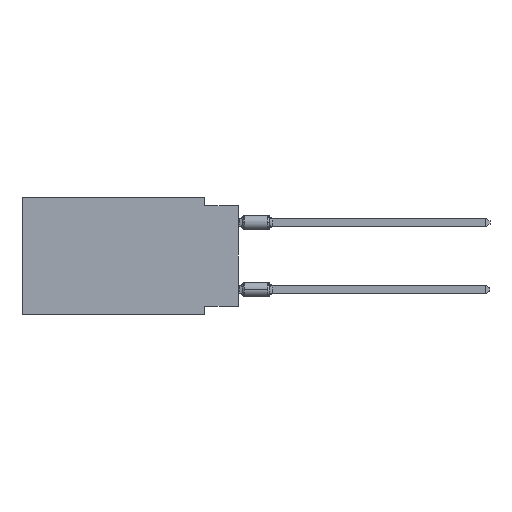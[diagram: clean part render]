
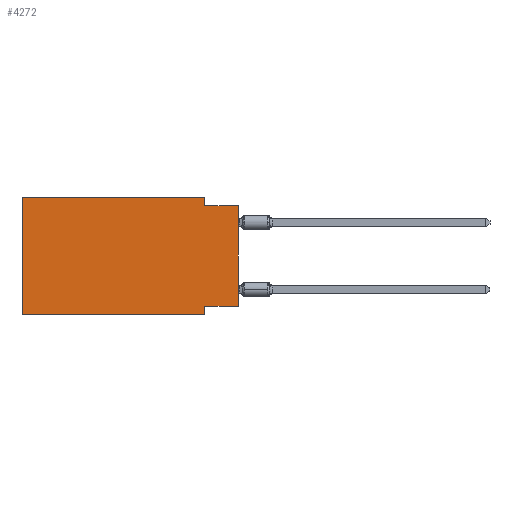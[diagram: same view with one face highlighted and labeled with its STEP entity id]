
A CAD part, left-side view. The second image highlights one B-rep face of the part: STEP entity #4272.
In plain terms, the highlighted planar face has unit normal (-1, 0, 0).
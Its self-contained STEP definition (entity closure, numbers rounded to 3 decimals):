
#333 = ORIENTED_EDGE ( 'NONE', *, *, #620, .F. ) ;
#569 = CARTESIAN_POINT ( 'NONE',  ( 0., 16.383, 0. ) ) ;
#620 = EDGE_CURVE ( 'NONE', #1620, #14196, #7437, .T. ) ;
#707 = CARTESIAN_POINT ( 'NONE',  ( 0., 2.54, -0.635 ) ) ;
#835 = LINE ( 'NONE', #14949, #6045 ) ;
#1177 = CARTESIAN_POINT ( 'NONE',  ( 0., 16.383, 0. ) ) ;
#1310 = CARTESIAN_POINT ( 'NONE',  ( 0., 2.54, 0. ) ) ;
#1328 = LINE ( 'NONE', #7187, #13705 ) ;
#1413 = ORIENTED_EDGE ( 'NONE', *, *, #7793, .F. ) ;
#1601 = VERTEX_POINT ( 'NONE', #569 ) ;
#1620 = VERTEX_POINT ( 'NONE', #16260 ) ;
#1751 = LINE ( 'NONE', #13072, #16311 ) ;
#1820 = EDGE_LOOP ( 'NONE', ( #7538, #10776, #17147, #4570, #17600, #7574, #1413, #333 ) ) ;
#2753 = VECTOR ( 'NONE', #13756, 1000. ) ;
#3415 = LINE ( 'NONE', #16224, #5672 ) ;
#3446 = CARTESIAN_POINT ( 'NONE',  ( 0., 0., -0.635 ) ) ;
#3975 = VERTEX_POINT ( 'NONE', #3446 ) ;
#4272 = ADVANCED_FACE ( 'NONE', ( #17069 ), #13265, .F. ) ;
#4570 = ORIENTED_EDGE ( 'NONE', *, *, #8958, .F. ) ;
#4643 = DIRECTION ( 'NONE',  ( 1., 0., 0. ) ) ;
#4846 = VERTEX_POINT ( 'NONE', #707 ) ;
#5672 = VECTOR ( 'NONE', #13625, 1000. ) ;
#6045 = VECTOR ( 'NONE', #14864, 1000. ) ;
#6121 = CARTESIAN_POINT ( 'NONE',  ( 0., 16.383, 0. ) ) ;
#6234 = VECTOR ( 'NONE', #6763, 1000. ) ;
#6477 = VECTOR ( 'NONE', #8734, 1000. ) ;
#6763 = DIRECTION ( 'NONE',  ( 0., -1., 0. ) ) ;
#7187 = CARTESIAN_POINT ( 'NONE',  ( 0., 2.54, -8.89 ) ) ;
#7432 = DIRECTION ( 'NONE',  ( 0., 0., -1. ) ) ;
#7437 = LINE ( 'NONE', #14387, #6477 ) ;
#7458 = VERTEX_POINT ( 'NONE', #8418 ) ;
#7538 = ORIENTED_EDGE ( 'NONE', *, *, #16291, .T. ) ;
#7574 = ORIENTED_EDGE ( 'NONE', *, *, #16974, .T. ) ;
#7793 = EDGE_CURVE ( 'NONE', #14196, #7458, #1328, .T. ) ;
#8112 = LINE ( 'NONE', #10788, #2753 ) ;
#8418 = CARTESIAN_POINT ( 'NONE',  ( 0., 2.54, -8.89 ) ) ;
#8717 = EDGE_CURVE ( 'NONE', #4846, #3975, #1751, .T. ) ;
#8734 = DIRECTION ( 'NONE',  ( 0., 1., 0. ) ) ;
#8958 = EDGE_CURVE ( 'NONE', #1601, #11495, #13986, .T. ) ;
#9048 = VECTOR ( 'NONE', #9551, 1000. ) ;
#9436 = VERTEX_POINT ( 'NONE', #18120 ) ;
#9551 = DIRECTION ( 'NONE',  ( 0., 0., 1. ) ) ;
#10027 = EDGE_CURVE ( 'NONE', #9436, #1601, #3415, .T. ) ;
#10159 = CARTESIAN_POINT ( 'NONE',  ( 0., 2.54, -8.255 ) ) ;
#10776 = ORIENTED_EDGE ( 'NONE', *, *, #8717, .F. ) ;
#10788 = CARTESIAN_POINT ( 'NONE',  ( 0., 16.383, -8.89 ) ) ;
#10926 = LINE ( 'NONE', #11024, #9048 ) ;
#11024 = CARTESIAN_POINT ( 'NONE',  ( 0., 0., 0. ) ) ;
#11495 = VERTEX_POINT ( 'NONE', #1310 ) ;
#13072 = CARTESIAN_POINT ( 'NONE',  ( 0., 0., -0.635 ) ) ;
#13265 = PLANE ( 'NONE',  #13297 ) ;
#13297 = AXIS2_PLACEMENT_3D ( 'NONE', #6121, #4643, #7432 ) ;
#13625 = DIRECTION ( 'NONE',  ( 0., 0., 1. ) ) ;
#13705 = VECTOR ( 'NONE', #18141, 1000. ) ;
#13756 = DIRECTION ( 'NONE',  ( 0., -1., 0. ) ) ;
#13986 = LINE ( 'NONE', #1177, #6234 ) ;
#14196 = VERTEX_POINT ( 'NONE', #10159 ) ;
#14387 = CARTESIAN_POINT ( 'NONE',  ( 0., 0., -8.255 ) ) ;
#14819 = EDGE_CURVE ( 'NONE', #11495, #4846, #835, .T. ) ;
#14864 = DIRECTION ( 'NONE',  ( 0., 0., -1. ) ) ;
#14949 = CARTESIAN_POINT ( 'NONE',  ( 0., 2.54, 0. ) ) ;
#15665 = DIRECTION ( 'NONE',  ( 0., -1., 0. ) ) ;
#16224 = CARTESIAN_POINT ( 'NONE',  ( 0., 16.383, 0. ) ) ;
#16260 = CARTESIAN_POINT ( 'NONE',  ( 0., 0., -8.255 ) ) ;
#16291 = EDGE_CURVE ( 'NONE', #1620, #3975, #10926, .T. ) ;
#16311 = VECTOR ( 'NONE', #15665, 1000. ) ;
#16974 = EDGE_CURVE ( 'NONE', #9436, #7458, #8112, .T. ) ;
#17069 = FACE_OUTER_BOUND ( 'NONE', #1820, .T. ) ;
#17147 = ORIENTED_EDGE ( 'NONE', *, *, #14819, .F. ) ;
#17600 = ORIENTED_EDGE ( 'NONE', *, *, #10027, .F. ) ;
#18120 = CARTESIAN_POINT ( 'NONE',  ( 0., 16.383, -8.89 ) ) ;
#18141 = DIRECTION ( 'NONE',  ( 0., 0., -1. ) ) ;
